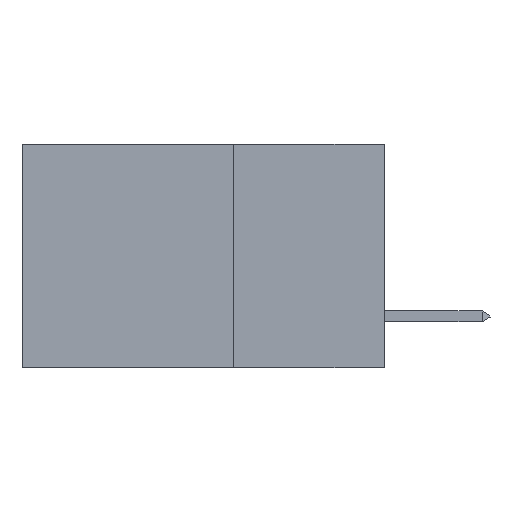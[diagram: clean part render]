
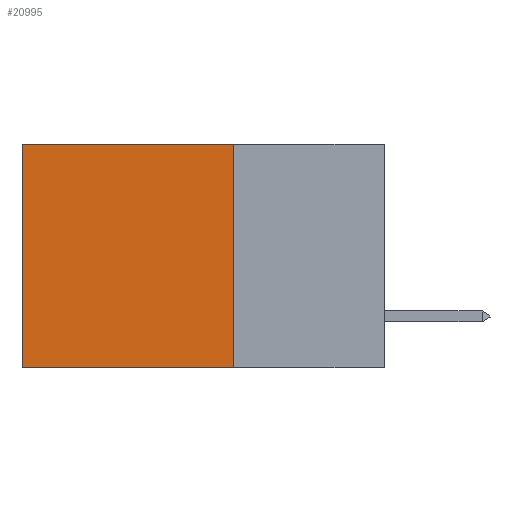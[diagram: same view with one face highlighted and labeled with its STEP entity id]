
A CAD part, left-side view. The second image highlights one B-rep face of the part: STEP entity #20995.
In plain terms, the highlighted planar face has unit normal (-1, 0, 0).
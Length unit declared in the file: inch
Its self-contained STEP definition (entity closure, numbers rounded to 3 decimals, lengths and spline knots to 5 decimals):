
#403 = CARTESIAN_POINT ( 'NONE',  ( 0.2875, 0.25, 0. ) ) ;
#2654 = EDGE_CURVE ( 'NONE', #16082, #13904, #29755, .T. ) ;
#4147 = ORIENTED_EDGE ( 'NONE', *, *, #31835, .F. ) ;
#5484 = VERTEX_POINT ( 'NONE', #28674 ) ;
#6776 = ORIENTED_EDGE ( 'NONE', *, *, #15311, .F. ) ;
#7158 = DIRECTION ( 'NONE',  ( 1., 0., 0. ) ) ;
#8116 = CARTESIAN_POINT ( 'NONE',  ( 0.2875, 0.25, 0. ) ) ;
#10390 = LINE ( 'NONE', #21757, #34820 ) ;
#11043 = ORIENTED_EDGE ( 'NONE', *, *, #40342, .T. ) ;
#11619 = DIRECTION ( 'NONE',  ( 0., 1., 0. ) ) ;
#11999 = LINE ( 'NONE', #35864, #12533 ) ;
#12533 = VECTOR ( 'NONE', #13609, 39.37008 ) ;
#13089 = CARTESIAN_POINT ( 'NONE',  ( 0.2875, 0.6, -0.37 ) ) ;
#13194 = AXIS2_PLACEMENT_3D ( 'NONE', #25085, #7158, #44859 ) ;
#13609 = DIRECTION ( 'NONE',  ( 0., 0., -1. ) ) ;
#13904 = VERTEX_POINT ( 'NONE', #13089 ) ;
#15311 = EDGE_CURVE ( 'NONE', #23367, #5484, #11999, .T. ) ;
#16082 = VERTEX_POINT ( 'NONE', #43650 ) ;
#19991 = FACE_OUTER_BOUND ( 'NONE', #27556, .T. ) ;
#20995 = ADVANCED_FACE ( 'NONE', ( #19991 ), #28930, .F. ) ;
#21757 = CARTESIAN_POINT ( 'NONE',  ( 0.2875, 0.25, -0.37 ) ) ;
#22558 = ORIENTED_EDGE ( 'NONE', *, *, #2654, .T. ) ;
#23367 = VERTEX_POINT ( 'NONE', #403 ) ;
#25085 = CARTESIAN_POINT ( 'NONE',  ( 0.2875, 0.25, 0. ) ) ;
#27556 = EDGE_LOOP ( 'NONE', ( #22558, #4147, #6776, #11043 ) ) ;
#28674 = CARTESIAN_POINT ( 'NONE',  ( 0.2875, 0.25, -0.37 ) ) ;
#28930 = PLANE ( 'NONE',  #13194 ) ;
#29755 = LINE ( 'NONE', #35780, #46861 ) ;
#31835 = EDGE_CURVE ( 'NONE', #5484, #13904, #10390, .T. ) ;
#34820 = VECTOR ( 'NONE', #36213, 39.37008 ) ;
#35780 = CARTESIAN_POINT ( 'NONE',  ( 0.2875, 0.6, 0. ) ) ;
#35864 = CARTESIAN_POINT ( 'NONE',  ( 0.2875, 0.25, 0. ) ) ;
#36213 = DIRECTION ( 'NONE',  ( 0., 1., 0. ) ) ;
#37383 = VECTOR ( 'NONE', #11619, 39.37008 ) ;
#37944 = LINE ( 'NONE', #8116, #37383 ) ;
#40342 = EDGE_CURVE ( 'NONE', #23367, #16082, #37944, .T. ) ;
#43650 = CARTESIAN_POINT ( 'NONE',  ( 0.2875, 0.6, 0. ) ) ;
#44093 = DIRECTION ( 'NONE',  ( 0., 0., -1. ) ) ;
#44859 = DIRECTION ( 'NONE',  ( 0., 0., -1. ) ) ;
#46861 = VECTOR ( 'NONE', #44093, 39.37008 ) ;
